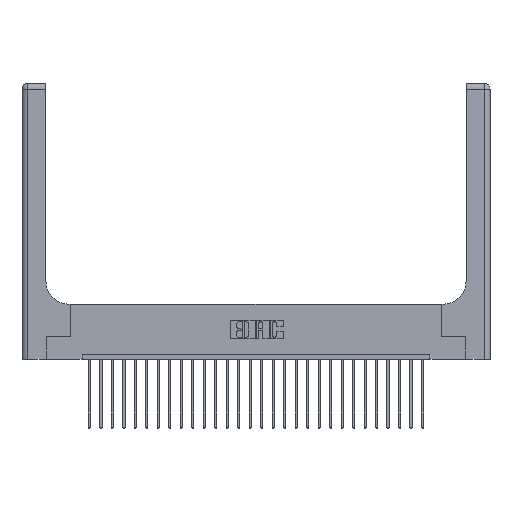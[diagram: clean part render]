
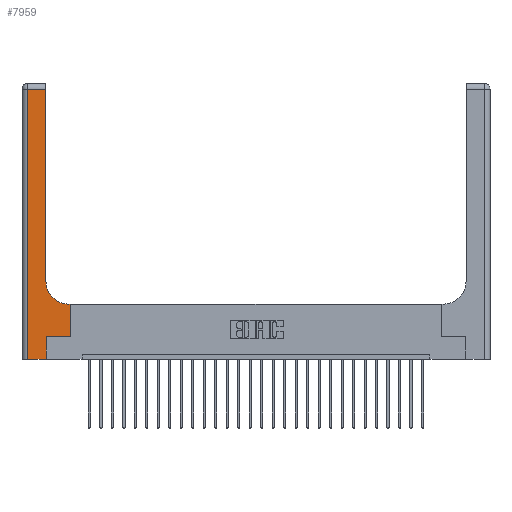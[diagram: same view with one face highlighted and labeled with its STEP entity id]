
A CAD part, top view. The second image highlights one B-rep face of the part: STEP entity #7959.
In plain terms, the highlighted planar face has unit normal (0, 0, 1).
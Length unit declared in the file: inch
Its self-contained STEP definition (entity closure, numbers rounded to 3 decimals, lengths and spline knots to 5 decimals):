
#483 = DIRECTION ( 'NONE',  ( 1., 0., 0. ) ) ;
#701 = CARTESIAN_POINT ( 'NONE',  ( 0.26, 2.94, 0.37 ) ) ;
#811 = DIRECTION ( 'NONE',  ( 0., 1., 0. ) ) ;
#1868 = EDGE_CURVE ( 'NONE', #4234, #17085, #23351, .T. ) ;
#2123 = VECTOR ( 'NONE', #483, 39.37008 ) ;
#2282 = CARTESIAN_POINT ( 'NONE',  ( 0.528, 0.25, 0.37 ) ) ;
#2363 = CARTESIAN_POINT ( 'NONE',  ( 0., 0., 0.37 ) ) ;
#2658 = DIRECTION ( 'NONE',  ( 1., 0., 0. ) ) ;
#2754 = ORIENTED_EDGE ( 'NONE', *, *, #15455, .T. ) ;
#4104 = CARTESIAN_POINT ( 'NONE',  ( 0.265, 0.25, 0.37 ) ) ;
#4234 = VERTEX_POINT ( 'NONE', #4104 ) ;
#4666 = CARTESIAN_POINT ( 'NONE',  ( 0.265, 0.25, 0.37 ) ) ;
#4895 = CARTESIAN_POINT ( 'NONE',  ( 0.06, 2.94, 0.37 ) ) ;
#4918 = ORIENTED_EDGE ( 'NONE', *, *, #20997, .T. ) ;
#5077 = DIRECTION ( 'NONE',  ( -1., 0., 0. ) ) ;
#5095 = LINE ( 'NONE', #18503, #17962 ) ;
#5424 = VERTEX_POINT ( 'NONE', #701 ) ;
#5984 = EDGE_CURVE ( 'NONE', #10592, #5424, #7793, .T. ) ;
#6048 = AXIS2_PLACEMENT_3D ( 'NONE', #16763, #6964, #25176 ) ;
#6053 = DIRECTION ( 'NONE',  ( 0., 1., 0. ) ) ;
#6257 = LINE ( 'NONE', #14279, #11825 ) ;
#6418 = LINE ( 'NONE', #2363, #2123 ) ;
#6964 = DIRECTION ( 'NONE',  ( 0., 0., -1. ) ) ;
#7083 = EDGE_LOOP ( 'NONE', ( #10469, #9534, #22850, #8918, #2754, #22982, #15291, #4918, #17052 ) ) ;
#7452 = VERTEX_POINT ( 'NONE', #4895 ) ;
#7793 = LINE ( 'NONE', #9263, #18505 ) ;
#7851 = EDGE_CURVE ( 'NONE', #7452, #22428, #6257, .T. ) ;
#7959 = ADVANCED_FACE ( 'NONE', ( #23397 ), #18670, .F. ) ;
#8006 = DIRECTION ( 'NONE',  ( 0., 1., 0. ) ) ;
#8598 = CARTESIAN_POINT ( 'NONE',  ( 0.528, 0.25, 0.37 ) ) ;
#8861 = DIRECTION ( 'NONE',  ( -1., 0., 0. ) ) ;
#8918 = ORIENTED_EDGE ( 'NONE', *, *, #10282, .T. ) ;
#9263 = CARTESIAN_POINT ( 'NONE',  ( 0.26, 3., 0.37 ) ) ;
#9534 = ORIENTED_EDGE ( 'NONE', *, *, #25256, .T. ) ;
#9565 = AXIS2_PLACEMENT_3D ( 'NONE', #12764, #24757, #5077 ) ;
#9993 = CARTESIAN_POINT ( 'NONE',  ( 0.26, 0.85, 0.37 ) ) ;
#10282 = EDGE_CURVE ( 'NONE', #22428, #20506, #6418, .T. ) ;
#10414 = VERTEX_POINT ( 'NONE', #22470 ) ;
#10469 = ORIENTED_EDGE ( 'NONE', *, *, #5984, .T. ) ;
#10592 = VERTEX_POINT ( 'NONE', #9993 ) ;
#11504 = EDGE_CURVE ( 'NONE', #22670, #10592, #22634, .T. ) ;
#11825 = VECTOR ( 'NONE', #24316, 39.37008 ) ;
#12195 = CARTESIAN_POINT ( 'NONE',  ( 0., 2.94, 0.37 ) ) ;
#12341 = VECTOR ( 'NONE', #8861, 39.37008 ) ;
#12764 = CARTESIAN_POINT ( 'NONE',  ( 0., 3., 0.37 ) ) ;
#14279 = CARTESIAN_POINT ( 'NONE',  ( 0.06, 3., 0.37 ) ) ;
#15116 = CARTESIAN_POINT ( 'NONE',  ( 0.06, 0., 0.37 ) ) ;
#15291 = ORIENTED_EDGE ( 'NONE', *, *, #16947, .T. ) ;
#15455 = EDGE_CURVE ( 'NONE', #20506, #4234, #5095, .T. ) ;
#16111 = VECTOR ( 'NONE', #22299, 39.37008 ) ;
#16684 = LINE ( 'NONE', #2282, #19365 ) ;
#16763 = CARTESIAN_POINT ( 'NONE',  ( 0.51, 0.85, 0.37 ) ) ;
#16947 = EDGE_CURVE ( 'NONE', #17085, #10414, #16684, .T. ) ;
#17052 = ORIENTED_EDGE ( 'NONE', *, *, #11504, .T. ) ;
#17085 = VERTEX_POINT ( 'NONE', #8598 ) ;
#17554 = VECTOR ( 'NONE', #2658, 39.37008 ) ;
#17962 = VECTOR ( 'NONE', #811, 39.37008 ) ;
#18503 = CARTESIAN_POINT ( 'NONE',  ( 0.265, 0., 0.37 ) ) ;
#18505 = VECTOR ( 'NONE', #8006, 39.37008 ) ;
#18670 = PLANE ( 'NONE',  #9565 ) ;
#18995 = LINE ( 'NONE', #20544, #12341 ) ;
#19117 = LINE ( 'NONE', #12195, #16111 ) ;
#19365 = VECTOR ( 'NONE', #6053, 39.37008 ) ;
#19614 = CARTESIAN_POINT ( 'NONE',  ( 0.51, 0.6, 0.37 ) ) ;
#20506 = VERTEX_POINT ( 'NONE', #23438 ) ;
#20544 = CARTESIAN_POINT ( 'NONE',  ( 0.26, 0.6, 0.37 ) ) ;
#20997 = EDGE_CURVE ( 'NONE', #10414, #22670, #18995, .T. ) ;
#22299 = DIRECTION ( 'NONE',  ( -1., 0., 0. ) ) ;
#22428 = VERTEX_POINT ( 'NONE', #15116 ) ;
#22470 = CARTESIAN_POINT ( 'NONE',  ( 0.528, 0.6, 0.37 ) ) ;
#22634 = CIRCLE ( 'NONE', #6048, 0.25 ) ;
#22670 = VERTEX_POINT ( 'NONE', #19614 ) ;
#22850 = ORIENTED_EDGE ( 'NONE', *, *, #7851, .T. ) ;
#22982 = ORIENTED_EDGE ( 'NONE', *, *, #1868, .T. ) ;
#23351 = LINE ( 'NONE', #4666, #17554 ) ;
#23397 = FACE_OUTER_BOUND ( 'NONE', #7083, .T. ) ;
#23438 = CARTESIAN_POINT ( 'NONE',  ( 0.265, 0., 0.37 ) ) ;
#24316 = DIRECTION ( 'NONE',  ( 0., -1., 0. ) ) ;
#24757 = DIRECTION ( 'NONE',  ( 0., 0., -1. ) ) ;
#25176 = DIRECTION ( 'NONE',  ( 1., 0., 0. ) ) ;
#25256 = EDGE_CURVE ( 'NONE', #5424, #7452, #19117, .T. ) ;
